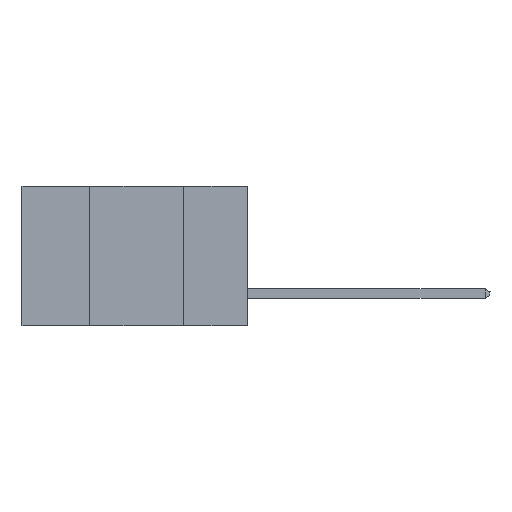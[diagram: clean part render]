
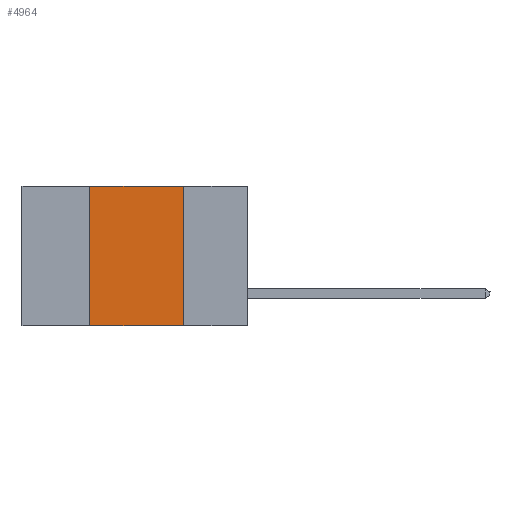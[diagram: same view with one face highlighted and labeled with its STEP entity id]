
A CAD part, left-side view. The second image highlights one B-rep face of the part: STEP entity #4964.
In plain terms, the highlighted planar face has unit normal (-1, 0, 0).
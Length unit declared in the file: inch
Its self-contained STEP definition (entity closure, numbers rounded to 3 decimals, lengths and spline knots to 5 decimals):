
#666 = VECTOR ( 'NONE', #9065, 39.37008 ) ;
#724 = EDGE_LOOP ( 'NONE', ( #5321, #8058, #5070, #1365 ) ) ;
#1053 = CARTESIAN_POINT ( 'NONE',  ( 0., 0.6, 0. ) ) ;
#1319 = CARTESIAN_POINT ( 'NONE',  ( 0., 0.42, 0. ) ) ;
#1365 = ORIENTED_EDGE ( 'NONE', *, *, #9619, .T. ) ;
#1763 = CARTESIAN_POINT ( 'NONE',  ( 0., 0.17, -0.37 ) ) ;
#1907 = VECTOR ( 'NONE', #7742, 39.37008 ) ;
#2025 = AXIS2_PLACEMENT_3D ( 'NONE', #5336, #3739, #8380 ) ;
#3032 = VECTOR ( 'NONE', #9371, 39.37008 ) ;
#3162 = DIRECTION ( 'NONE',  ( 0., 0., 1. ) ) ;
#3739 = DIRECTION ( 'NONE',  ( 1., 0., 0. ) ) ;
#3854 = CARTESIAN_POINT ( 'NONE',  ( 0., 0.17, -0.37 ) ) ;
#4078 = VECTOR ( 'NONE', #3162, 39.37008 ) ;
#4964 = ADVANCED_FACE ( 'NONE', ( #5277 ), #6265, .F. ) ;
#4980 = EDGE_CURVE ( 'NONE', #6135, #11493, #8445, .T. ) ;
#5070 = ORIENTED_EDGE ( 'NONE', *, *, #9887, .F. ) ;
#5277 = FACE_OUTER_BOUND ( 'NONE', #724, .T. ) ;
#5321 = ORIENTED_EDGE ( 'NONE', *, *, #4980, .F. ) ;
#5336 = CARTESIAN_POINT ( 'NONE',  ( 0., 0.6, 0. ) ) ;
#5771 = CARTESIAN_POINT ( 'NONE',  ( 0., 0.42, -0.37 ) ) ;
#5813 = LINE ( 'NONE', #1053, #1907 ) ;
#6135 = VERTEX_POINT ( 'NONE', #10252 ) ;
#6265 = PLANE ( 'NONE',  #2025 ) ;
#7742 = DIRECTION ( 'NONE',  ( 0., -1., 0. ) ) ;
#7764 = CARTESIAN_POINT ( 'NONE',  ( 0., 0.42, -0.37 ) ) ;
#8058 = ORIENTED_EDGE ( 'NONE', *, *, #12062, .F. ) ;
#8380 = DIRECTION ( 'NONE',  ( 0., 0., -1. ) ) ;
#8445 = LINE ( 'NONE', #1763, #3032 ) ;
#8957 = VERTEX_POINT ( 'NONE', #1319 ) ;
#9065 = DIRECTION ( 'NONE',  ( 0., -1., 0. ) ) ;
#9317 = VERTEX_POINT ( 'NONE', #5771 ) ;
#9371 = DIRECTION ( 'NONE',  ( 0., 0., -1. ) ) ;
#9619 = EDGE_CURVE ( 'NONE', #9317, #11493, #12082, .T. ) ;
#9887 = EDGE_CURVE ( 'NONE', #9317, #8957, #11630, .T. ) ;
#10252 = CARTESIAN_POINT ( 'NONE',  ( 0., 0.17, 0. ) ) ;
#11220 = CARTESIAN_POINT ( 'NONE',  ( 0., 0.6, -0.37 ) ) ;
#11493 = VERTEX_POINT ( 'NONE', #3854 ) ;
#11630 = LINE ( 'NONE', #7764, #4078 ) ;
#12062 = EDGE_CURVE ( 'NONE', #8957, #6135, #5813, .T. ) ;
#12082 = LINE ( 'NONE', #11220, #666 ) ;
